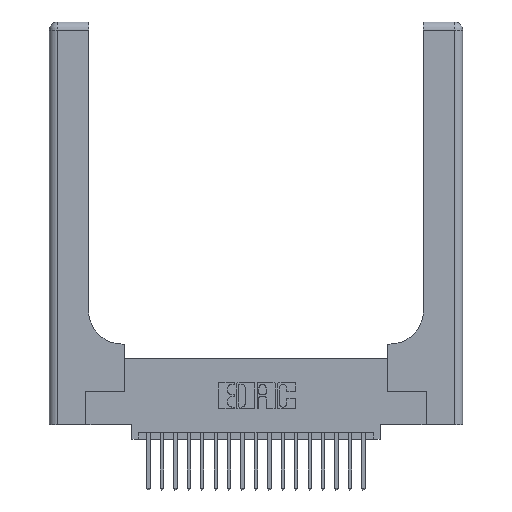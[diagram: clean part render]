
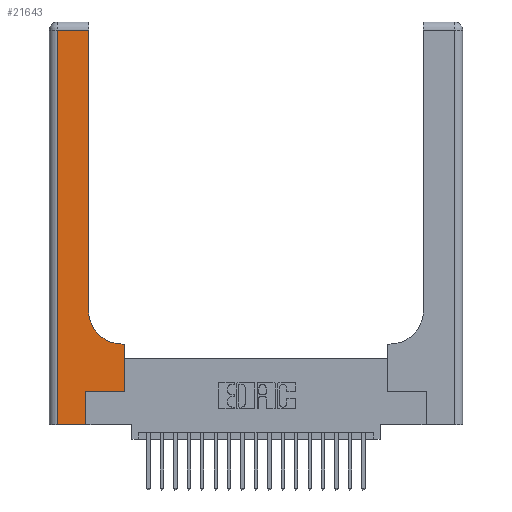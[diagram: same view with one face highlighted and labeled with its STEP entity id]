
A CAD part, top view. The second image highlights one B-rep face of the part: STEP entity #21643.
In plain terms, the highlighted planar face has unit normal (0, 0, 1).
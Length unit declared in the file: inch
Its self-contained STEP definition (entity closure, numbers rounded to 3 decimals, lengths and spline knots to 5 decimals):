
#307 = ORIENTED_EDGE ( 'NONE', *, *, #9594, .T. ) ;
#399 = CARTESIAN_POINT ( 'NONE',  ( 0.2915, 3., 0.37 ) ) ;
#475 = CARTESIAN_POINT ( 'NONE',  ( 0.06, 0., 0.37 ) ) ;
#574 = CIRCLE ( 'NONE', #1826, 0.25 ) ;
#677 = VECTOR ( 'NONE', #3063, 39.37008 ) ;
#980 = LINE ( 'NONE', #4668, #14613 ) ;
#1244 = FACE_OUTER_BOUND ( 'NONE', #9984, .T. ) ;
#1379 = ORIENTED_EDGE ( 'NONE', *, *, #5951, .T. ) ;
#1826 = AXIS2_PLACEMENT_3D ( 'NONE', #12674, #2398, #14365 ) ;
#2398 = DIRECTION ( 'NONE',  ( 0., 0., -1. ) ) ;
#2442 = PLANE ( 'NONE',  #4192 ) ;
#2897 = LINE ( 'NONE', #10075, #20478 ) ;
#2972 = CARTESIAN_POINT ( 'NONE',  ( 0.269, 0., 0.37 ) ) ;
#3063 = DIRECTION ( 'NONE',  ( 0., 1., 0. ) ) ;
#3240 = ORIENTED_EDGE ( 'NONE', *, *, #9430, .T. ) ;
#3266 = EDGE_CURVE ( 'NONE', #17336, #20039, #2897, .T. ) ;
#3272 = DIRECTION ( 'NONE',  ( 0., -1., 0. ) ) ;
#3347 = LINE ( 'NONE', #13537, #13007 ) ;
#3496 = CARTESIAN_POINT ( 'NONE',  ( 0., 2.94, 0.37 ) ) ;
#3634 = VECTOR ( 'NONE', #15180, 39.37008 ) ;
#3774 = ORIENTED_EDGE ( 'NONE', *, *, #3266, .T. ) ;
#4192 = AXIS2_PLACEMENT_3D ( 'NONE', #16107, #5876, #17806 ) ;
#4306 = ORIENTED_EDGE ( 'NONE', *, *, #21853, .T. ) ;
#4668 = CARTESIAN_POINT ( 'NONE',  ( 0.269, 0.25, 0.37 ) ) ;
#5205 = LINE ( 'NONE', #15011, #677 ) ;
#5210 = CARTESIAN_POINT ( 'NONE',  ( 0.5585, 0.6, 0.37 ) ) ;
#5819 = EDGE_CURVE ( 'NONE', #8194, #12186, #20827, .T. ) ;
#5876 = DIRECTION ( 'NONE',  ( 0., 0., -1. ) ) ;
#5951 = EDGE_CURVE ( 'NONE', #11636, #8194, #574, .T. ) ;
#7134 = LINE ( 'NONE', #11366, #16200 ) ;
#7612 = VERTEX_POINT ( 'NONE', #5210 ) ;
#7686 = LINE ( 'NONE', #20287, #3634 ) ;
#8194 = VERTEX_POINT ( 'NONE', #12091 ) ;
#8350 = DIRECTION ( 'NONE',  ( 1., 0., 0. ) ) ;
#8368 = VERTEX_POINT ( 'NONE', #14238 ) ;
#8449 = VERTEX_POINT ( 'NONE', #12766 ) ;
#8718 = EDGE_CURVE ( 'NONE', #20039, #8449, #7686, .T. ) ;
#9430 = EDGE_CURVE ( 'NONE', #13046, #17336, #3347, .T. ) ;
#9594 = EDGE_CURVE ( 'NONE', #8368, #7612, #5205, .T. ) ;
#9984 = EDGE_LOOP ( 'NONE', ( #20299, #16337, #3240, #3774, #12902, #4306, #307, #13946, #1379 ) ) ;
#10075 = CARTESIAN_POINT ( 'NONE',  ( 0., 0., 0.37 ) ) ;
#10648 = DIRECTION ( 'NONE',  ( 0., 1., 0. ) ) ;
#11184 = VECTOR ( 'NONE', #13756, 39.37008 ) ;
#11366 = CARTESIAN_POINT ( 'NONE',  ( 0.2915, 0.6, 0.37 ) ) ;
#11636 = VERTEX_POINT ( 'NONE', #19069 ) ;
#12091 = CARTESIAN_POINT ( 'NONE',  ( 0.2915, 0.85, 0.37 ) ) ;
#12186 = VERTEX_POINT ( 'NONE', #17499 ) ;
#12674 = CARTESIAN_POINT ( 'NONE',  ( 0.5415, 0.85, 0.37 ) ) ;
#12766 = CARTESIAN_POINT ( 'NONE',  ( 0.269, 0.25, 0.37 ) ) ;
#12902 = ORIENTED_EDGE ( 'NONE', *, *, #8718, .T. ) ;
#13007 = VECTOR ( 'NONE', #3272, 39.37008 ) ;
#13046 = VERTEX_POINT ( 'NONE', #21047 ) ;
#13537 = CARTESIAN_POINT ( 'NONE',  ( 0.06, 3., 0.37 ) ) ;
#13756 = DIRECTION ( 'NONE',  ( -1., 0., 0. ) ) ;
#13946 = ORIENTED_EDGE ( 'NONE', *, *, #21784, .T. ) ;
#13977 = EDGE_CURVE ( 'NONE', #12186, #13046, #19660, .T. ) ;
#14238 = CARTESIAN_POINT ( 'NONE',  ( 0.5585, 0.25, 0.37 ) ) ;
#14365 = DIRECTION ( 'NONE',  ( 1., 0., 0. ) ) ;
#14613 = VECTOR ( 'NONE', #16618, 39.37008 ) ;
#15011 = CARTESIAN_POINT ( 'NONE',  ( 0.5585, 0.25, 0.37 ) ) ;
#15180 = DIRECTION ( 'NONE',  ( 0., 1., 0. ) ) ;
#15800 = VECTOR ( 'NONE', #10648, 39.37008 ) ;
#16107 = CARTESIAN_POINT ( 'NONE',  ( 0., 3., 0.37 ) ) ;
#16200 = VECTOR ( 'NONE', #21500, 39.37008 ) ;
#16337 = ORIENTED_EDGE ( 'NONE', *, *, #13977, .T. ) ;
#16618 = DIRECTION ( 'NONE',  ( 1., 0., 0. ) ) ;
#17336 = VERTEX_POINT ( 'NONE', #475 ) ;
#17499 = CARTESIAN_POINT ( 'NONE',  ( 0.2915, 2.94, 0.37 ) ) ;
#17806 = DIRECTION ( 'NONE',  ( -1., 0., 0. ) ) ;
#19069 = CARTESIAN_POINT ( 'NONE',  ( 0.5415, 0.6, 0.37 ) ) ;
#19660 = LINE ( 'NONE', #3496, #11184 ) ;
#20039 = VERTEX_POINT ( 'NONE', #2972 ) ;
#20287 = CARTESIAN_POINT ( 'NONE',  ( 0.269, 0., 0.37 ) ) ;
#20299 = ORIENTED_EDGE ( 'NONE', *, *, #5819, .T. ) ;
#20478 = VECTOR ( 'NONE', #8350, 39.37008 ) ;
#20827 = LINE ( 'NONE', #399, #15800 ) ;
#21047 = CARTESIAN_POINT ( 'NONE',  ( 0.06, 2.94, 0.37 ) ) ;
#21500 = DIRECTION ( 'NONE',  ( -1., 0., 0. ) ) ;
#21643 = ADVANCED_FACE ( 'NONE', ( #1244 ), #2442, .F. ) ;
#21784 = EDGE_CURVE ( 'NONE', #7612, #11636, #7134, .T. ) ;
#21853 = EDGE_CURVE ( 'NONE', #8449, #8368, #980, .T. ) ;
